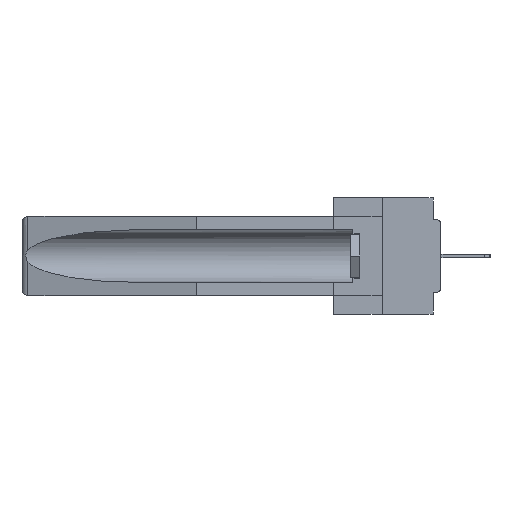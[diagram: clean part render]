
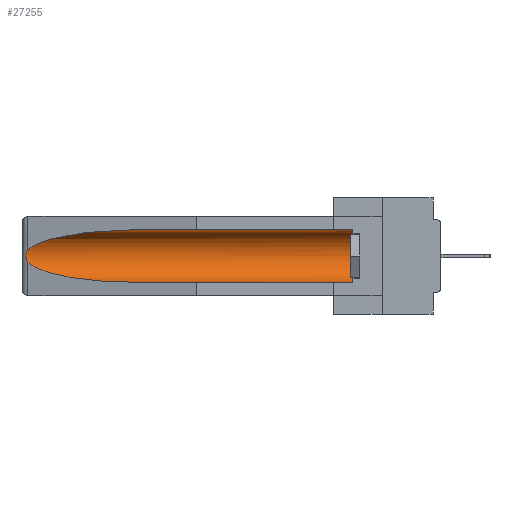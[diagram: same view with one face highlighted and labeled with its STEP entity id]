
A CAD part, left-side view. The second image highlights one B-rep face of the part: STEP entity #27255.
In plain terms, the highlighted cylindrical face has radius 2.857 mm (diameter 5.715 mm), a partial arc.
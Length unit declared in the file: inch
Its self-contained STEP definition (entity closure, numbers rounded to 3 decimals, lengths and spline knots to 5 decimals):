
#265 = CARTESIAN_POINT ( 'NONE',  ( 0.155, 1.07973, -0.284 ) ) ;
#488 = CARTESIAN_POINT ( 'NONE',  ( 0.26537, 1.52718, -0.19328 ) ) ;
#890 = LINE ( 'NONE', #12048, #1278 ) ;
#1126 = CARTESIAN_POINT ( 'NONE',  ( 0.155, 0.126, -0.1715 ) ) ;
#1278 = VECTOR ( 'NONE', #35089, 39.37008 ) ;
#1299 = VERTEX_POINT ( 'NONE', #25622 ) ;
#1392 = CARTESIAN_POINT ( 'NONE',  ( 0.26655, 1.53094, -0.18657 ) ) ;
#1969 = LINE ( 'NONE', #35992, #20029 ) ;
#3320 = CARTESIAN_POINT ( 'NONE',  ( 0.155, -0.30754, -0.1715 ) ) ;
#3648 = CARTESIAN_POINT ( 'NONE',  ( 0.25451, 1.48313, -0.24835 ) ) ;
#3746 = VERTEX_POINT ( 'NONE', #25919 ) ;
#4572 =( BOUNDED_CURVE ( )  B_SPLINE_CURVE ( 3, ( #26751, #32346, #6881, #29900 ),
 .UNSPECIFIED., .F., .F. ) 
 B_SPLINE_CURVE_WITH_KNOTS ( ( 4, 4 ),
 ( 4.71239, 6.08839 ),
 .UNSPECIFIED. ) 
 CURVE ( )  GEOMETRIC_REPRESENTATION_ITEM ( )  RATIONAL_B_SPLINE_CURVE ( ( 1., 0.848, 0.848, 1. ) ) 
 REPRESENTATION_ITEM ( '' )  );
#4643 = CARTESIAN_POINT ( 'NONE',  ( 0.26537, 1.52718, -0.19328 ) ) ;
#5301 = AXIS2_PLACEMENT_3D ( 'NONE', #3320, #14828, #17787 ) ;
#5418 = VERTEX_POINT ( 'NONE', #7706 ) ;
#5779 = ORIENTED_EDGE ( 'NONE', *, *, #29962, .T. ) ;
#6133 = CARTESIAN_POINT ( 'NONE',  ( 0.155, 1.07973, -0.059 ) ) ;
#6190 = VERTEX_POINT ( 'NONE', #4643 ) ;
#6463 = VERTEX_POINT ( 'NONE', #6133 ) ;
#6881 = CARTESIAN_POINT ( 'NONE',  ( 0.25451, 1.48313, -0.09465 ) ) ;
#7141 = CARTESIAN_POINT ( 'NONE',  ( 0.2673, 1.53269, -0.17917 ) ) ;
#7706 = CARTESIAN_POINT ( 'NONE',  ( 0.26537, 1.52718, -0.14972 ) ) ;
#8674 = EDGE_LOOP ( 'NONE', ( #10981, #24342, #12654, #9913, #5779, #15468 ) ) ;
#9760 = CARTESIAN_POINT ( 'NONE',  ( 0.2675, 1.53308, -0.16763 ) ) ;
#9913 = ORIENTED_EDGE ( 'NONE', *, *, #15481, .F. ) ;
#9933 = CARTESIAN_POINT ( 'NONE',  ( 0.2675, 1.53308, -0.17534 ) ) ;
#10518 = DIRECTION ( 'NONE',  ( 0., 1., 0. ) ) ;
#10610 = FACE_OUTER_BOUND ( 'NONE', #8674, .T. ) ;
#10693 = EDGE_CURVE ( 'NONE', #6463, #5418, #4572, .T. ) ;
#10981 = ORIENTED_EDGE ( 'NONE', *, *, #10693, .T. ) ;
#12048 = CARTESIAN_POINT ( 'NONE',  ( 0.155, -0.30754, -0.284 ) ) ;
#12287 = B_SPLINE_CURVE_WITH_KNOTS ( 'NONE', 3,
 ( #28889, #35031, #35403, #20901, #9760, #9933, #7141, #1392, #18264, #27019 ),
 .UNSPECIFIED., .F., .F.,
 ( 4, 2, 2, 2, 4 ),
 ( 0., 0.00029, 0.00058, 0.00087, 0.00117 ),
 .UNSPECIFIED. ) ;
#12654 = ORIENTED_EDGE ( 'NONE', *, *, #30269, .T. ) ;
#12675 = EDGE_CURVE ( 'NONE', #5418, #6190, #12287, .T. ) ;
#14254 = CARTESIAN_POINT ( 'NONE',  ( 0.21114, 1.30732, -0.284 ) ) ;
#14828 = DIRECTION ( 'NONE',  ( 0., 1., 0. ) ) ;
#14880 = CIRCLE ( 'NONE', #31500, 0.1125 ) ;
#15468 = ORIENTED_EDGE ( 'NONE', *, *, #23150, .T. ) ;
#15481 = EDGE_CURVE ( 'NONE', #3746, #25463, #890, .T. ) ;
#17438 = CYLINDRICAL_SURFACE ( 'NONE', #5301, 0.1125 ) ;
#17787 = DIRECTION ( 'NONE',  ( 0., 0., 1. ) ) ;
#18036 = DIRECTION ( 'NONE',  ( 0., 0., 1. ) ) ;
#18264 = CARTESIAN_POINT ( 'NONE',  ( 0.26597, 1.5296, -0.19026 ) ) ;
#20029 = VECTOR ( 'NONE', #10518, 39.37008 ) ;
#20901 = CARTESIAN_POINT ( 'NONE',  ( 0.2673, 1.5327, -0.16383 ) ) ;
#23150 = EDGE_CURVE ( 'NONE', #1299, #6463, #1969, .T. ) ;
#23512 = CARTESIAN_POINT ( 'NONE',  ( 0.155, 1.07973, -0.284 ) ) ;
#23792 = DIRECTION ( 'NONE',  ( 0., -1., 0. ) ) ;
#24342 = ORIENTED_EDGE ( 'NONE', *, *, #12675, .T. ) ;
#25463 = VERTEX_POINT ( 'NONE', #265 ) ;
#25622 = CARTESIAN_POINT ( 'NONE',  ( 0.155, 0.126, -0.059 ) ) ;
#25919 = CARTESIAN_POINT ( 'NONE',  ( 0.155, 0.126, -0.284 ) ) ;
#26751 = CARTESIAN_POINT ( 'NONE',  ( 0.155, 1.07973, -0.059 ) ) ;
#27019 = CARTESIAN_POINT ( 'NONE',  ( 0.26537, 1.52718, -0.19328 ) ) ;
#27255 = ADVANCED_FACE ( 'NONE', ( #10610 ), #17438, .F. ) ;
#28889 = CARTESIAN_POINT ( 'NONE',  ( 0.26537, 1.52718, -0.14972 ) ) ;
#29900 = CARTESIAN_POINT ( 'NONE',  ( 0.26537, 1.52718, -0.14972 ) ) ;
#29962 = EDGE_CURVE ( 'NONE', #3746, #1299, #14880, .T. ) ;
#30269 = EDGE_CURVE ( 'NONE', #6190, #25463, #32801, .T. ) ;
#31500 = AXIS2_PLACEMENT_3D ( 'NONE', #1126, #23792, #18036 ) ;
#32346 = CARTESIAN_POINT ( 'NONE',  ( 0.21114, 1.30732, -0.059 ) ) ;
#32801 =( BOUNDED_CURVE ( )  B_SPLINE_CURVE ( 3, ( #488, #3648, #14254, #23512 ),
 .UNSPECIFIED., .F., .T. ) 
 B_SPLINE_CURVE_WITH_KNOTS ( ( 4, 4 ),
 ( 0.1948, 1.5708 ),
 .UNSPECIFIED. ) 
 CURVE ( )  GEOMETRIC_REPRESENTATION_ITEM ( )  RATIONAL_B_SPLINE_CURVE ( ( 1., 0.848, 0.848, 1. ) ) 
 REPRESENTATION_ITEM ( '' )  );
#35031 = CARTESIAN_POINT ( 'NONE',  ( 0.26597, 1.52961, -0.15275 ) ) ;
#35089 = DIRECTION ( 'NONE',  ( 0., 1., 0. ) ) ;
#35403 = CARTESIAN_POINT ( 'NONE',  ( 0.26654, 1.53092, -0.15636 ) ) ;
#35992 = CARTESIAN_POINT ( 'NONE',  ( 0.155, -0.30754, -0.059 ) ) ;
